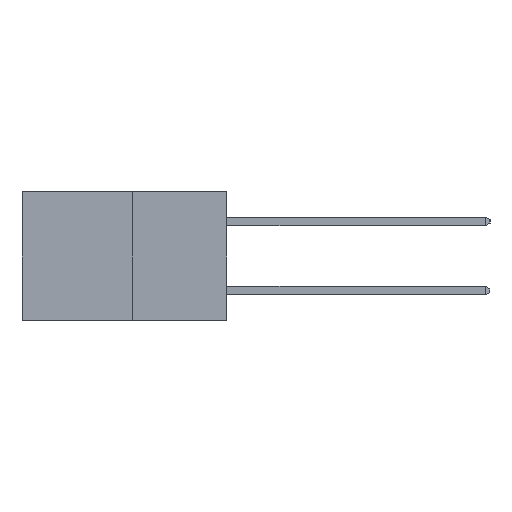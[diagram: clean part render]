
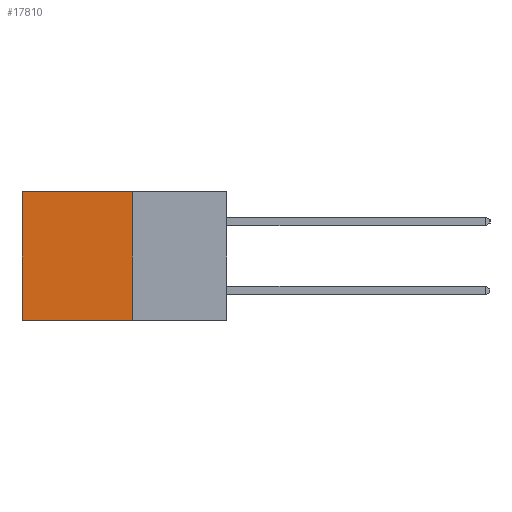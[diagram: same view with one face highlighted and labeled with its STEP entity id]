
A CAD part, left-side view. The second image highlights one B-rep face of the part: STEP entity #17810.
In plain terms, the highlighted planar face has unit normal (-1, 0, 0).
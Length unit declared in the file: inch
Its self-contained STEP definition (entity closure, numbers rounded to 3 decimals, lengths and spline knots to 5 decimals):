
#1535 = PLANE ( 'NONE',  #10234 ) ;
#2170 = EDGE_CURVE ( 'NONE', #3175, #18602, #4914, .T. ) ;
#2304 = CARTESIAN_POINT ( 'NONE',  ( 0.277, 0.27, 0. ) ) ;
#3175 = VERTEX_POINT ( 'NONE', #7575 ) ;
#3943 = DIRECTION ( 'NONE',  ( 0., 0., -1. ) ) ;
#4914 = LINE ( 'NONE', #28592, #29245 ) ;
#5347 = CARTESIAN_POINT ( 'NONE',  ( 0.277, 0.27, -0.37 ) ) ;
#5873 = DIRECTION ( 'NONE',  ( 0., 0., -1. ) ) ;
#7247 = DIRECTION ( 'NONE',  ( 0., 1., 0. ) ) ;
#7575 = CARTESIAN_POINT ( 'NONE',  ( 0.277, 0.59, 0. ) ) ;
#9862 = ORIENTED_EDGE ( 'NONE', *, *, #23830, .F. ) ;
#10205 = CARTESIAN_POINT ( 'NONE',  ( 0.277, 0.27, 0. ) ) ;
#10234 = AXIS2_PLACEMENT_3D ( 'NONE', #22869, #18241, #3943 ) ;
#10811 = VECTOR ( 'NONE', #28300, 39.37008 ) ;
#11535 = EDGE_CURVE ( 'NONE', #19860, #18602, #13633, .T. ) ;
#12881 = VECTOR ( 'NONE', #7247, 39.37008 ) ;
#13633 = LINE ( 'NONE', #21539, #12881 ) ;
#14738 = LINE ( 'NONE', #17884, #20362 ) ;
#14740 = ORIENTED_EDGE ( 'NONE', *, *, #2170, .T. ) ;
#17614 = ORIENTED_EDGE ( 'NONE', *, *, #26544, .T. ) ;
#17810 = ADVANCED_FACE ( 'NONE', ( #26987 ), #1535, .F. ) ;
#17884 = CARTESIAN_POINT ( 'NONE',  ( 0.277, 0.27, -0.37 ) ) ;
#18045 = ORIENTED_EDGE ( 'NONE', *, *, #11535, .F. ) ;
#18241 = DIRECTION ( 'NONE',  ( 1., 0., 0. ) ) ;
#18602 = VERTEX_POINT ( 'NONE', #29924 ) ;
#19860 = VERTEX_POINT ( 'NONE', #5347 ) ;
#20362 = VECTOR ( 'NONE', #5873, 39.37008 ) ;
#21539 = CARTESIAN_POINT ( 'NONE',  ( 0.277, 0.27, -0.37 ) ) ;
#22869 = CARTESIAN_POINT ( 'NONE',  ( 0.277, 0.27, -0.37 ) ) ;
#23830 = EDGE_CURVE ( 'NONE', #27388, #19860, #14738, .T. ) ;
#25890 = EDGE_LOOP ( 'NONE', ( #14740, #18045, #9862, #17614 ) ) ;
#26544 = EDGE_CURVE ( 'NONE', #27388, #3175, #28815, .T. ) ;
#26987 = FACE_OUTER_BOUND ( 'NONE', #25890, .T. ) ;
#27388 = VERTEX_POINT ( 'NONE', #10205 ) ;
#28300 = DIRECTION ( 'NONE',  ( 0., 1., 0. ) ) ;
#28592 = CARTESIAN_POINT ( 'NONE',  ( 0.277, 0.59, -0.37 ) ) ;
#28664 = DIRECTION ( 'NONE',  ( 0., 0., -1. ) ) ;
#28815 = LINE ( 'NONE', #2304, #10811 ) ;
#29245 = VECTOR ( 'NONE', #28664, 39.37008 ) ;
#29924 = CARTESIAN_POINT ( 'NONE',  ( 0.277, 0.59, -0.37 ) ) ;
